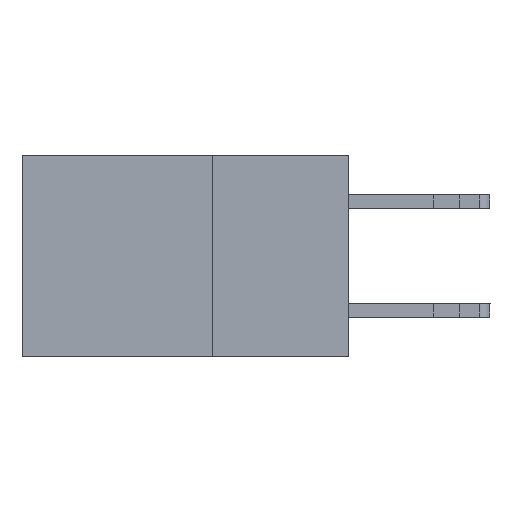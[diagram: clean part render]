
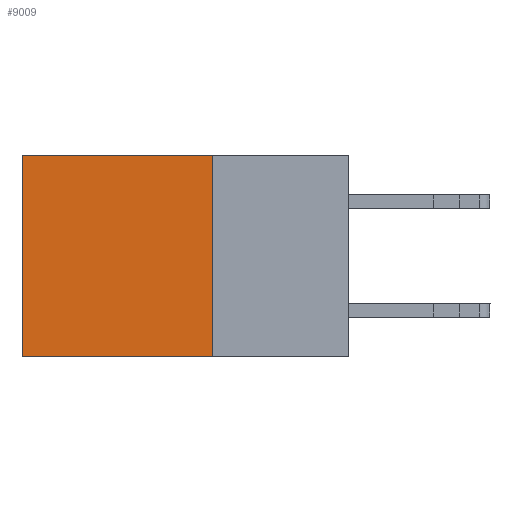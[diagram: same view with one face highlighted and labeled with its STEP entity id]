
A CAD part, left-side view. The second image highlights one B-rep face of the part: STEP entity #9009.
In plain terms, the highlighted planar face has unit normal (-1, 0, 0).
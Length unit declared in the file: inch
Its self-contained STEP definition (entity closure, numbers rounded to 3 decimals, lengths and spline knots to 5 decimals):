
#595 = DIRECTION ( 'NONE',  ( 0., 1., 0. ) ) ;
#657 = CARTESIAN_POINT ( 'NONE',  ( 0.298, 0.25, -0.37 ) ) ;
#2542 = VERTEX_POINT ( 'NONE', #13990 ) ;
#2766 = CARTESIAN_POINT ( 'NONE',  ( 0.298, 0.6, 0. ) ) ;
#2974 = VECTOR ( 'NONE', #6414, 39.37008 ) ;
#3231 = EDGE_CURVE ( 'NONE', #2542, #11647, #13503, .T. ) ;
#4205 = DIRECTION ( 'NONE',  ( 1., 0., 0. ) ) ;
#4576 = EDGE_LOOP ( 'NONE', ( #7845, #12244, #7053, #13203 ) ) ;
#5260 = DIRECTION ( 'NONE',  ( 0., 0., -1. ) ) ;
#5417 = CARTESIAN_POINT ( 'NONE',  ( 0.298, 0.25, 0. ) ) ;
#6414 = DIRECTION ( 'NONE',  ( 0., 0., -1. ) ) ;
#6415 = CARTESIAN_POINT ( 'NONE',  ( 0.298, 0.6, -0.37 ) ) ;
#6831 = EDGE_CURVE ( 'NONE', #12609, #7821, #15062, .T. ) ;
#7053 = ORIENTED_EDGE ( 'NONE', *, *, #15137, .F. ) ;
#7257 = AXIS2_PLACEMENT_3D ( 'NONE', #14139, #4205, #15618 ) ;
#7615 = CARTESIAN_POINT ( 'NONE',  ( 0.298, 0.25, 0. ) ) ;
#7821 = VERTEX_POINT ( 'NONE', #14992 ) ;
#7845 = ORIENTED_EDGE ( 'NONE', *, *, #14958, .T. ) ;
#7995 = CARTESIAN_POINT ( 'NONE',  ( 0.298, 0.25, 0. ) ) ;
#8067 = LINE ( 'NONE', #7615, #2974 ) ;
#9009 = ADVANCED_FACE ( 'NONE', ( #11189 ), #12863, .F. ) ;
#10568 = DIRECTION ( 'NONE',  ( 0., 1., 0. ) ) ;
#11189 = FACE_OUTER_BOUND ( 'NONE', #4576, .T. ) ;
#11647 = VERTEX_POINT ( 'NONE', #6415 ) ;
#12244 = ORIENTED_EDGE ( 'NONE', *, *, #3231, .F. ) ;
#12501 = VECTOR ( 'NONE', #10568, 39.37008 ) ;
#12609 = VERTEX_POINT ( 'NONE', #5417 ) ;
#12863 = PLANE ( 'NONE',  #7257 ) ;
#13203 = ORIENTED_EDGE ( 'NONE', *, *, #6831, .T. ) ;
#13297 = LINE ( 'NONE', #2766, #15257 ) ;
#13503 = LINE ( 'NONE', #657, #15475 ) ;
#13990 = CARTESIAN_POINT ( 'NONE',  ( 0.298, 0.25, -0.37 ) ) ;
#14139 = CARTESIAN_POINT ( 'NONE',  ( 0.298, 0.25, 0. ) ) ;
#14958 = EDGE_CURVE ( 'NONE', #7821, #11647, #13297, .T. ) ;
#14992 = CARTESIAN_POINT ( 'NONE',  ( 0.298, 0.6, 0. ) ) ;
#15062 = LINE ( 'NONE', #7995, #12501 ) ;
#15137 = EDGE_CURVE ( 'NONE', #12609, #2542, #8067, .T. ) ;
#15257 = VECTOR ( 'NONE', #5260, 39.37008 ) ;
#15475 = VECTOR ( 'NONE', #595, 39.37008 ) ;
#15618 = DIRECTION ( 'NONE',  ( 0., 0., -1. ) ) ;
